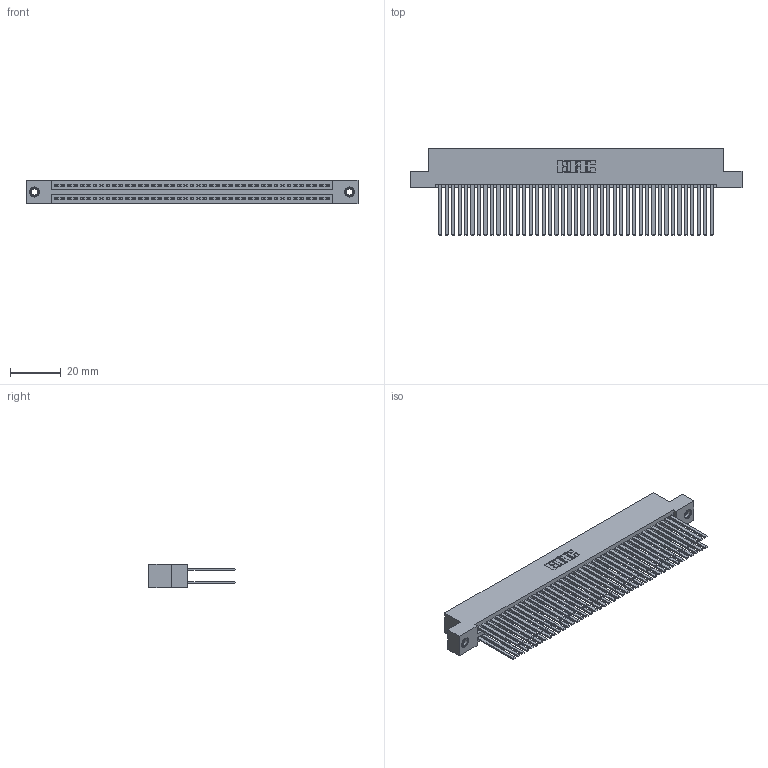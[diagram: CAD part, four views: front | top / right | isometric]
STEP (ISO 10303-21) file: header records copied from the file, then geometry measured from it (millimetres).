
FILE_DESCRIPTION (( 'STEP AP203' ), '1' );
FILE_NAME ('395-086-544-207.STEP', '2018-11-28T21:30:15', ( '' ), ( '' ), 'SwSTEP 2.0', 'SolidWorks 2016', '' );
FILE_SCHEMA (( 'CONFIG_CONTROL_DESIGN' ));
Length unit declared in the file: inch
Products named in the file (4): 345-292-001_345-293-144; 345-250-001_345-250-005-103; 345 Part_Flush Mounting Lugs - 0.156 Dia-TI; 395-086-544-207
Assembly tree (89 placements, depth 2):
  395-086-544-207
    345 Part_Flush Mounting Lugs - 0.156 Dia-TI
    345-292-001_345-293-144  x86
    345-250-001_345-250-005-103  x2
Bounding box: 130.43 x 33.96 x 9.4 mm (x, y, z)
Volume: 13871.3 mm3; surface area: 24084.8 mm2
Topology: 89 solids, 89 shells, 3970 faces, 11743 edges, 7706 vertices
Faces by surface type: plane 2606, cylinder 1348, cone 12, torus 4
Entity records: 34606 total; most frequent: CARTESIAN_POINT 5779, ORIENTED_EDGE 5706, DIRECTION 5119, EDGE_CURVE 2853, LINE 2533, VECTOR 2533, VERTEX_POINT 1896, AXIS2_PLACEMENT_3D 1293
